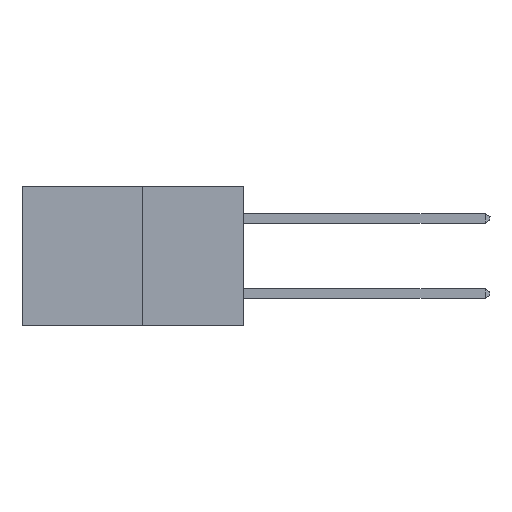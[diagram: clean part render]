
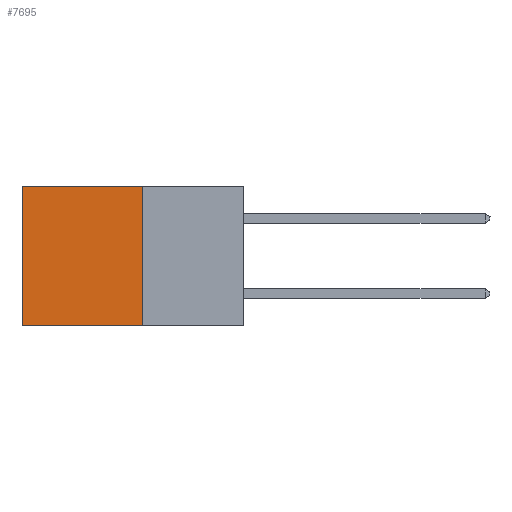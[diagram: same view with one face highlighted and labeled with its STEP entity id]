
A CAD part, left-side view. The second image highlights one B-rep face of the part: STEP entity #7695.
In plain terms, the highlighted planar face has unit normal (-1, 0, 0).
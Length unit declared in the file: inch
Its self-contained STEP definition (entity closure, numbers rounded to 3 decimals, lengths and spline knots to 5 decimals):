
#462 = VECTOR ( 'NONE', #11744, 39.37008 ) ;
#5277 = LINE ( 'NONE', #25960, #462 ) ;
#6026 = VERTEX_POINT ( 'NONE', #12981 ) ;
#6419 = VECTOR ( 'NONE', #11504, 39.37008 ) ;
#7695 = ADVANCED_FACE ( 'NONE', ( #17401 ), #22499, .F. ) ;
#8754 = EDGE_LOOP ( 'NONE', ( #19343, #9120, #14550, #19956 ) ) ;
#9120 = ORIENTED_EDGE ( 'NONE', *, *, #17259, .F. ) ;
#11326 = LINE ( 'NONE', #25398, #16746 ) ;
#11504 = DIRECTION ( 'NONE',  ( 0., 0., -1. ) ) ;
#11744 = DIRECTION ( 'NONE',  ( 0., 0., -1. ) ) ;
#12497 = EDGE_CURVE ( 'NONE', #6026, #15190, #5277, .T. ) ;
#12790 = CARTESIAN_POINT ( 'NONE',  ( 0.277, 0.27, -0.37 ) ) ;
#12981 = CARTESIAN_POINT ( 'NONE',  ( 0.277, 0.59, 0. ) ) ;
#13143 = DIRECTION ( 'NONE',  ( 0., 1., 0. ) ) ;
#14550 = ORIENTED_EDGE ( 'NONE', *, *, #15844, .F. ) ;
#14825 = VERTEX_POINT ( 'NONE', #12790 ) ;
#14938 = EDGE_CURVE ( 'NONE', #16300, #6026, #11326, .T. ) ;
#15190 = VERTEX_POINT ( 'NONE', #24044 ) ;
#15844 = EDGE_CURVE ( 'NONE', #16300, #14825, #22104, .T. ) ;
#16178 = AXIS2_PLACEMENT_3D ( 'NONE', #23434, #22490, #22429 ) ;
#16300 = VERTEX_POINT ( 'NONE', #25234 ) ;
#16746 = VECTOR ( 'NONE', #13143, 39.37008 ) ;
#17259 = EDGE_CURVE ( 'NONE', #14825, #15190, #23949, .T. ) ;
#17401 = FACE_OUTER_BOUND ( 'NONE', #8754, .T. ) ;
#17679 = CARTESIAN_POINT ( 'NONE',  ( 0.277, 0.27, -0.37 ) ) ;
#19343 = ORIENTED_EDGE ( 'NONE', *, *, #12497, .T. ) ;
#19956 = ORIENTED_EDGE ( 'NONE', *, *, #14938, .T. ) ;
#21315 = CARTESIAN_POINT ( 'NONE',  ( 0.277, 0.27, -0.37 ) ) ;
#22104 = LINE ( 'NONE', #17679, #6419 ) ;
#22429 = DIRECTION ( 'NONE',  ( 0., 0., -1. ) ) ;
#22490 = DIRECTION ( 'NONE',  ( 1., 0., 0. ) ) ;
#22499 = PLANE ( 'NONE',  #16178 ) ;
#22634 = VECTOR ( 'NONE', #23386, 39.37008 ) ;
#23386 = DIRECTION ( 'NONE',  ( 0., 1., 0. ) ) ;
#23434 = CARTESIAN_POINT ( 'NONE',  ( 0.277, 0.27, -0.37 ) ) ;
#23949 = LINE ( 'NONE', #21315, #22634 ) ;
#24044 = CARTESIAN_POINT ( 'NONE',  ( 0.277, 0.59, -0.37 ) ) ;
#25234 = CARTESIAN_POINT ( 'NONE',  ( 0.277, 0.27, 0. ) ) ;
#25398 = CARTESIAN_POINT ( 'NONE',  ( 0.277, 0.27, 0. ) ) ;
#25960 = CARTESIAN_POINT ( 'NONE',  ( 0.277, 0.59, -0.37 ) ) ;
